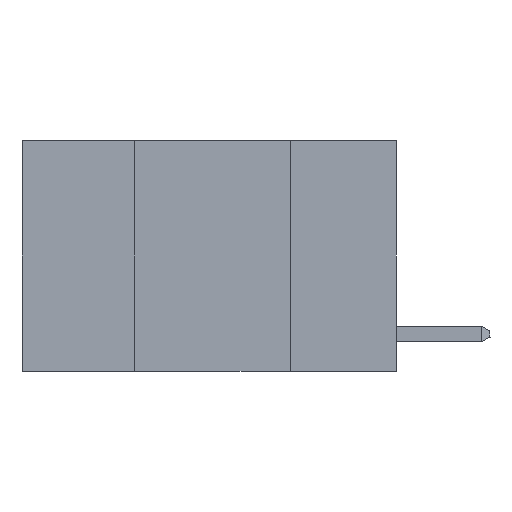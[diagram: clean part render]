
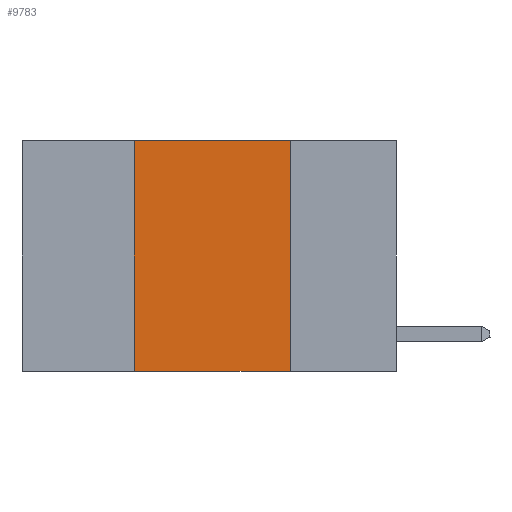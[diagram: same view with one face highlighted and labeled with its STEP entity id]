
A CAD part, left-side view. The second image highlights one B-rep face of the part: STEP entity #9783.
In plain terms, the highlighted planar face has unit normal (-1, 0, 0).
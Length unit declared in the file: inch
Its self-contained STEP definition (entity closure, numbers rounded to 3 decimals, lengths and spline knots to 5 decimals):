
#95 = VECTOR ( 'NONE', #4115, 39.37008 ) ;
#100 = CARTESIAN_POINT ( 'NONE',  ( 0., 0.17, 0. ) ) ;
#190 = ORIENTED_EDGE ( 'NONE', *, *, #5460, .F. ) ;
#729 = VERTEX_POINT ( 'NONE', #15568 ) ;
#1552 = CARTESIAN_POINT ( 'NONE',  ( 0., 0.6, 0. ) ) ;
#1842 = CARTESIAN_POINT ( 'NONE',  ( 0., 0.42, 0. ) ) ;
#1941 = LINE ( 'NONE', #1552, #12775 ) ;
#2253 = CARTESIAN_POINT ( 'NONE',  ( 0., 0.6, 0. ) ) ;
#2258 = EDGE_CURVE ( 'NONE', #7403, #16619, #7542, .T. ) ;
#3311 = CARTESIAN_POINT ( 'NONE',  ( 0., 0.42, 0. ) ) ;
#3707 = DIRECTION ( 'NONE',  ( 1., 0., 0. ) ) ;
#4075 = LINE ( 'NONE', #15896, #95 ) ;
#4115 = DIRECTION ( 'NONE',  ( 0., -1., 0. ) ) ;
#4223 = EDGE_CURVE ( 'NONE', #16239, #7403, #1941, .T. ) ;
#4457 = ORIENTED_EDGE ( 'NONE', *, *, #4223, .F. ) ;
#5460 = EDGE_CURVE ( 'NONE', #729, #16239, #11702, .T. ) ;
#7403 = VERTEX_POINT ( 'NONE', #100 ) ;
#7542 = LINE ( 'NONE', #11995, #17001 ) ;
#8733 = ORIENTED_EDGE ( 'NONE', *, *, #2258, .F. ) ;
#9783 = ADVANCED_FACE ( 'NONE', ( #12329 ), #10433, .F. ) ;
#9849 = AXIS2_PLACEMENT_3D ( 'NONE', #2253, #3707, #13057 ) ;
#10433 = PLANE ( 'NONE',  #9849 ) ;
#11164 = DIRECTION ( 'NONE',  ( 0., -1., 0. ) ) ;
#11702 = LINE ( 'NONE', #1842, #15878 ) ;
#11940 = DIRECTION ( 'NONE',  ( 0., 0., -1. ) ) ;
#11995 = CARTESIAN_POINT ( 'NONE',  ( 0., 0.17, 0. ) ) ;
#12329 = FACE_OUTER_BOUND ( 'NONE', #13228, .T. ) ;
#12722 = DIRECTION ( 'NONE',  ( 0., 0., 1. ) ) ;
#12775 = VECTOR ( 'NONE', #11164, 39.37008 ) ;
#13057 = DIRECTION ( 'NONE',  ( 0., 0., -1. ) ) ;
#13228 = EDGE_LOOP ( 'NONE', ( #8733, #4457, #190, #17259 ) ) ;
#13416 = CARTESIAN_POINT ( 'NONE',  ( 0., 0.17, -0.37 ) ) ;
#15235 = EDGE_CURVE ( 'NONE', #729, #16619, #4075, .T. ) ;
#15568 = CARTESIAN_POINT ( 'NONE',  ( 0., 0.42, -0.37 ) ) ;
#15878 = VECTOR ( 'NONE', #12722, 39.37008 ) ;
#15896 = CARTESIAN_POINT ( 'NONE',  ( 0., 0.6, -0.37 ) ) ;
#16239 = VERTEX_POINT ( 'NONE', #3311 ) ;
#16619 = VERTEX_POINT ( 'NONE', #13416 ) ;
#17001 = VECTOR ( 'NONE', #11940, 39.37008 ) ;
#17259 = ORIENTED_EDGE ( 'NONE', *, *, #15235, .T. ) ;
